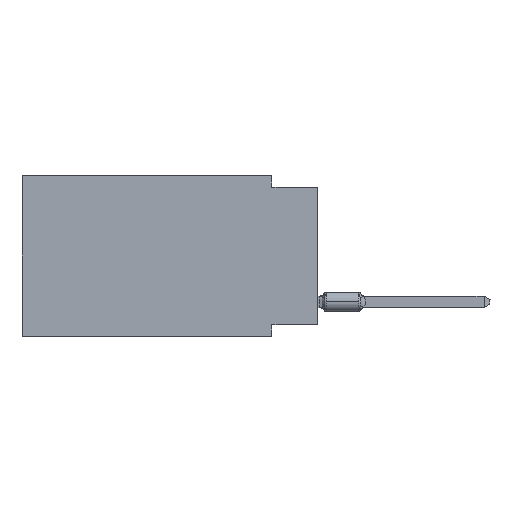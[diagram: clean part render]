
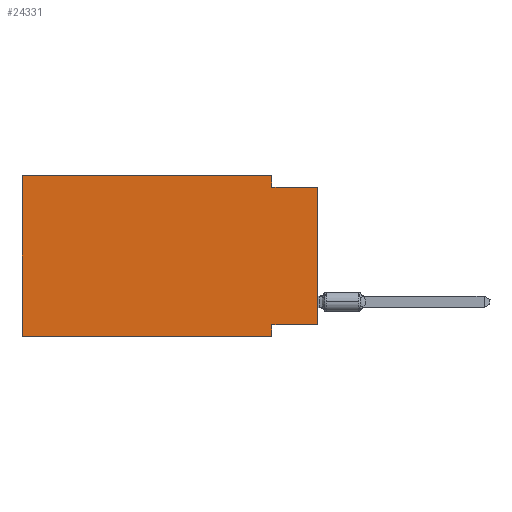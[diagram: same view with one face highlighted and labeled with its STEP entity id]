
A CAD part, left-side view. The second image highlights one B-rep face of the part: STEP entity #24331.
In plain terms, the highlighted planar face has unit normal (-1, 0, 0).
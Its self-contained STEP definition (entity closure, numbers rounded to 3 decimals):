
#40 = CARTESIAN_POINT ( 'NONE',  ( 0., 16.383, 0. ) ) ;
#428 = EDGE_CURVE ( 'NONE', #15625, #18455, #24997, .T. ) ;
#1592 = VERTEX_POINT ( 'NONE', #30012 ) ;
#2139 = EDGE_CURVE ( 'NONE', #18908, #3735, #16050, .T. ) ;
#3735 = VERTEX_POINT ( 'NONE', #12841 ) ;
#3838 = VERTEX_POINT ( 'NONE', #14316 ) ;
#4264 = EDGE_CURVE ( 'NONE', #3838, #18908, #5728, .T. ) ;
#4749 = DIRECTION ( 'NONE',  ( 0., 0., -1. ) ) ;
#5462 = EDGE_LOOP ( 'NONE', ( #13966, #19193, #33830, #5511, #19585, #22303, #28513, #14943 ) ) ;
#5511 = ORIENTED_EDGE ( 'NONE', *, *, #2139, .F. ) ;
#5517 = VECTOR ( 'NONE', #12880, 1000. ) ;
#5728 = LINE ( 'NONE', #40, #6052 ) ;
#5882 = AXIS2_PLACEMENT_3D ( 'NONE', #13089, #30958, #12742 ) ;
#5998 = VECTOR ( 'NONE', #23665, 1000. ) ;
#6052 = VECTOR ( 'NONE', #33843, 1000. ) ;
#6054 = LINE ( 'NONE', #29076, #11162 ) ;
#6775 = CARTESIAN_POINT ( 'NONE',  ( 0., 16.383, 0. ) ) ;
#7461 = CARTESIAN_POINT ( 'NONE',  ( 0., 16.383, 0. ) ) ;
#8523 = DIRECTION ( 'NONE',  ( 0., 1., 0. ) ) ;
#9707 = LINE ( 'NONE', #24352, #21961 ) ;
#10541 = CARTESIAN_POINT ( 'NONE',  ( 0., 0., 0. ) ) ;
#10603 = PLANE ( 'NONE',  #5882 ) ;
#11162 = VECTOR ( 'NONE', #8523, 1000. ) ;
#11522 = VECTOR ( 'NONE', #4749, 1000. ) ;
#11845 = CARTESIAN_POINT ( 'NONE',  ( 0., 2.54, -0.635 ) ) ;
#12742 = DIRECTION ( 'NONE',  ( 0., 0., -1. ) ) ;
#12823 = EDGE_CURVE ( 'NONE', #3838, #33434, #24483, .T. ) ;
#12841 = CARTESIAN_POINT ( 'NONE',  ( 0., 2.54, 0. ) ) ;
#12880 = DIRECTION ( 'NONE',  ( 0., -1., 0. ) ) ;
#13089 = CARTESIAN_POINT ( 'NONE',  ( 0., 16.383, 0. ) ) ;
#13966 = ORIENTED_EDGE ( 'NONE', *, *, #428, .T. ) ;
#14316 = CARTESIAN_POINT ( 'NONE',  ( 0., 16.383, -8.89 ) ) ;
#14943 = ORIENTED_EDGE ( 'NONE', *, *, #33312, .F. ) ;
#15625 = VERTEX_POINT ( 'NONE', #27594 ) ;
#15729 = CARTESIAN_POINT ( 'NONE',  ( 0., 16.383, -8.89 ) ) ;
#15777 = FACE_OUTER_BOUND ( 'NONE', #5462, .T. ) ;
#16050 = LINE ( 'NONE', #6775, #24759 ) ;
#17577 = CARTESIAN_POINT ( 'NONE',  ( 0., 2.54, 0. ) ) ;
#18379 = DIRECTION ( 'NONE',  ( 0., -1., 0. ) ) ;
#18455 = VERTEX_POINT ( 'NONE', #24741 ) ;
#18908 = VERTEX_POINT ( 'NONE', #7461 ) ;
#19193 = ORIENTED_EDGE ( 'NONE', *, *, #30647, .F. ) ;
#19585 = ORIENTED_EDGE ( 'NONE', *, *, #4264, .F. ) ;
#20834 = LINE ( 'NONE', #17577, #5998 ) ;
#21634 = EDGE_CURVE ( 'NONE', #1592, #33434, #30789, .T. ) ;
#21961 = VECTOR ( 'NONE', #27394, 1000. ) ;
#22303 = ORIENTED_EDGE ( 'NONE', *, *, #12823, .T. ) ;
#23665 = DIRECTION ( 'NONE',  ( 0., 0., -1. ) ) ;
#23766 = VERTEX_POINT ( 'NONE', #11845 ) ;
#23861 = DIRECTION ( 'NONE',  ( 0., 0., 1. ) ) ;
#24331 = ADVANCED_FACE ( 'NONE', ( #15777 ), #10603, .F. ) ;
#24352 = CARTESIAN_POINT ( 'NONE',  ( 0., 0., -0.635 ) ) ;
#24483 = LINE ( 'NONE', #15729, #5517 ) ;
#24741 = CARTESIAN_POINT ( 'NONE',  ( 0., 0., -0.635 ) ) ;
#24759 = VECTOR ( 'NONE', #18379, 1000. ) ;
#24997 = LINE ( 'NONE', #10541, #32183 ) ;
#26135 = EDGE_CURVE ( 'NONE', #3735, #23766, #20834, .T. ) ;
#27394 = DIRECTION ( 'NONE',  ( 0., -1., 0. ) ) ;
#27530 = CARTESIAN_POINT ( 'NONE',  ( 0., 2.54, -8.89 ) ) ;
#27594 = CARTESIAN_POINT ( 'NONE',  ( 0., 0., -8.255 ) ) ;
#28513 = ORIENTED_EDGE ( 'NONE', *, *, #21634, .F. ) ;
#29076 = CARTESIAN_POINT ( 'NONE',  ( 0., 0., -8.255 ) ) ;
#30012 = CARTESIAN_POINT ( 'NONE',  ( 0., 2.54, -8.255 ) ) ;
#30647 = EDGE_CURVE ( 'NONE', #23766, #18455, #9707, .T. ) ;
#30789 = LINE ( 'NONE', #36293, #11522 ) ;
#30958 = DIRECTION ( 'NONE',  ( 1., 0., 0. ) ) ;
#32183 = VECTOR ( 'NONE', #23861, 1000. ) ;
#33312 = EDGE_CURVE ( 'NONE', #15625, #1592, #6054, .T. ) ;
#33434 = VERTEX_POINT ( 'NONE', #27530 ) ;
#33830 = ORIENTED_EDGE ( 'NONE', *, *, #26135, .F. ) ;
#33843 = DIRECTION ( 'NONE',  ( 0., 0., 1. ) ) ;
#36293 = CARTESIAN_POINT ( 'NONE',  ( 0., 2.54, -8.89 ) ) ;
